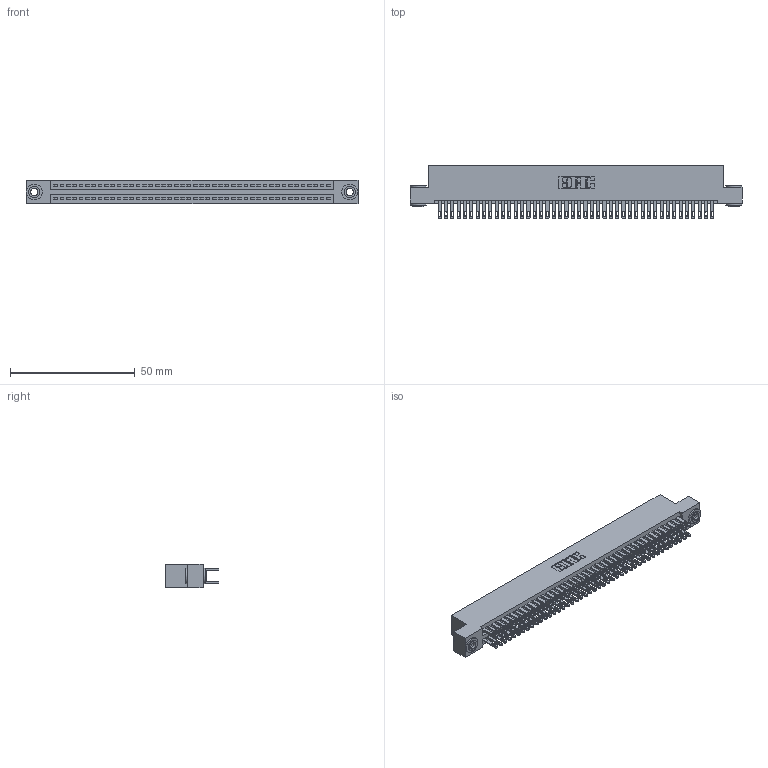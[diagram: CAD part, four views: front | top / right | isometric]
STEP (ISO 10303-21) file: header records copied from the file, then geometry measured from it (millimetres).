
FILE_DESCRIPTION (( 'STEP AP203' ), '1' );
FILE_NAME ('345-088-500-203.STEP', '2019-11-01T09:52:01', ( '' ), ( '' ), 'SwSTEP 2.0', 'SolidWorks 2016', '' );
FILE_SCHEMA (( 'CONFIG_CONTROL_DESIGN' ));
Length unit declared in the file: inch
Products named in the file (4): 345-088-500-203; 345-250-002_345-250-002-102; 345-292-001_345-293-100; 345 Part_Flush Mounting Lugs - 0.156 Dia-TH
Assembly tree (91 placements, depth 2):
  345-088-500-203
    345 Part_Flush Mounting Lugs - 0.156 Dia-TH
    345-292-001_345-293-100  x88
    345-250-002_345-250-002-102  x2
Bounding box: 132.97 x 21.51 x 9.4 mm (x, y, z)
Volume: 13223.6 mm3; surface area: 20687.9 mm2
Topology: 91 solids, 91 shells, 4212 faces, 12825 edges, 8546 vertices
Faces by surface type: plane 2466, cylinder 1738, cone 8
Entity records: 34834 total; most frequent: CARTESIAN_POINT 5811, ORIENTED_EDGE 5738, DIRECTION 5155, EDGE_CURVE 2869, VECTOR 2533, LINE 2533, VERTEX_POINT 1910, AXIS2_PLACEMENT_3D 1311
